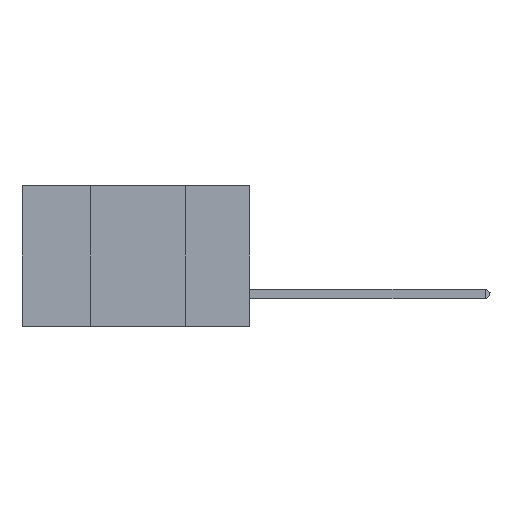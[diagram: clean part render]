
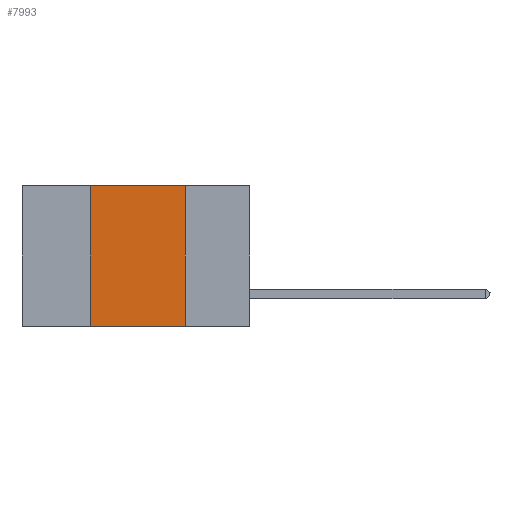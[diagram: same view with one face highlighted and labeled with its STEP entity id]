
A CAD part, left-side view. The second image highlights one B-rep face of the part: STEP entity #7993.
In plain terms, the highlighted planar face has unit normal (-1, 0, 0).
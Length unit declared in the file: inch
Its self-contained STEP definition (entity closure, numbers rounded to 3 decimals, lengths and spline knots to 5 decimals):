
#196 = LINE ( 'NONE', #1935, #16939 ) ;
#997 = CARTESIAN_POINT ( 'NONE',  ( 0., 0.17, 0. ) ) ;
#1125 = LINE ( 'NONE', #11857, #8141 ) ;
#1935 = CARTESIAN_POINT ( 'NONE',  ( 0., 0.42, 0. ) ) ;
#2338 = DIRECTION ( 'NONE',  ( 1., 0., 0. ) ) ;
#3130 = EDGE_CURVE ( 'NONE', #16307, #8393, #1125, .T. ) ;
#3999 = EDGE_CURVE ( 'NONE', #16307, #7661, #196, .T. ) ;
#4036 = CARTESIAN_POINT ( 'NONE',  ( 0., 0.6, 0. ) ) ;
#6046 = EDGE_CURVE ( 'NONE', #7661, #7921, #13452, .T. ) ;
#6497 = DIRECTION ( 'NONE',  ( 0., -1., 0. ) ) ;
#7661 = VERTEX_POINT ( 'NONE', #15501 ) ;
#7921 = VERTEX_POINT ( 'NONE', #997 ) ;
#7953 = VECTOR ( 'NONE', #13608, 39.37008 ) ;
#7993 = ADVANCED_FACE ( 'NONE', ( #12119 ), #15830, .F. ) ;
#8141 = VECTOR ( 'NONE', #6497, 39.37008 ) ;
#8272 = VECTOR ( 'NONE', #17382, 39.37008 ) ;
#8393 = VERTEX_POINT ( 'NONE', #8529 ) ;
#8529 = CARTESIAN_POINT ( 'NONE',  ( 0., 0.17, -0.37 ) ) ;
#8722 = CARTESIAN_POINT ( 'NONE',  ( 0., 0.42, -0.37 ) ) ;
#9159 = ORIENTED_EDGE ( 'NONE', *, *, #3999, .F. ) ;
#9982 = ORIENTED_EDGE ( 'NONE', *, *, #10275, .F. ) ;
#10275 = EDGE_CURVE ( 'NONE', #7921, #8393, #11875, .T. ) ;
#10390 = CARTESIAN_POINT ( 'NONE',  ( 0., 0.17, 0. ) ) ;
#11857 = CARTESIAN_POINT ( 'NONE',  ( 0., 0.6, -0.37 ) ) ;
#11875 = LINE ( 'NONE', #10390, #8272 ) ;
#12119 = FACE_OUTER_BOUND ( 'NONE', #17012, .T. ) ;
#13400 = CARTESIAN_POINT ( 'NONE',  ( 0., 0.6, 0. ) ) ;
#13452 = LINE ( 'NONE', #4036, #7953 ) ;
#13608 = DIRECTION ( 'NONE',  ( 0., -1., 0. ) ) ;
#14136 = DIRECTION ( 'NONE',  ( 0., 0., 1. ) ) ;
#14536 = DIRECTION ( 'NONE',  ( 0., 0., -1. ) ) ;
#15501 = CARTESIAN_POINT ( 'NONE',  ( 0., 0.42, 0. ) ) ;
#15626 = AXIS2_PLACEMENT_3D ( 'NONE', #13400, #2338, #14536 ) ;
#15830 = PLANE ( 'NONE',  #15626 ) ;
#16307 = VERTEX_POINT ( 'NONE', #8722 ) ;
#16384 = ORIENTED_EDGE ( 'NONE', *, *, #6046, .F. ) ;
#16531 = ORIENTED_EDGE ( 'NONE', *, *, #3130, .T. ) ;
#16939 = VECTOR ( 'NONE', #14136, 39.37008 ) ;
#17012 = EDGE_LOOP ( 'NONE', ( #9982, #16384, #9159, #16531 ) ) ;
#17382 = DIRECTION ( 'NONE',  ( 0., 0., -1. ) ) ;
